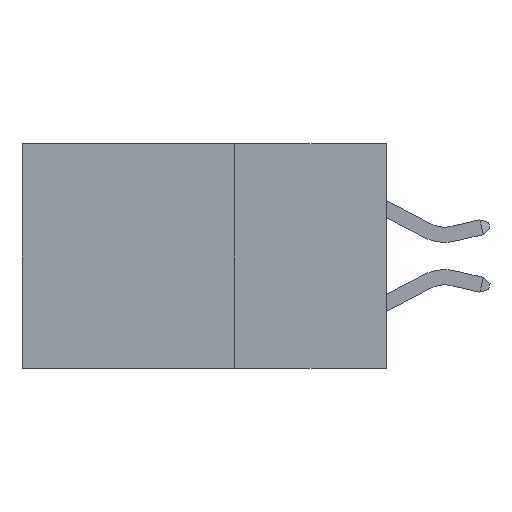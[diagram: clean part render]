
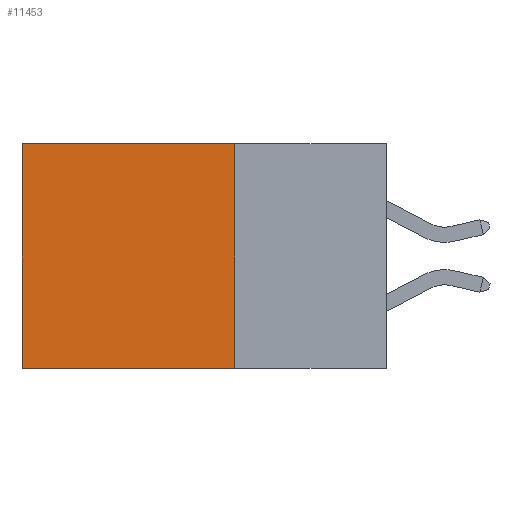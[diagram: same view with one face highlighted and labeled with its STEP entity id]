
A CAD part, left-side view. The second image highlights one B-rep face of the part: STEP entity #11453.
In plain terms, the highlighted planar face has unit normal (-1, 0, 0).
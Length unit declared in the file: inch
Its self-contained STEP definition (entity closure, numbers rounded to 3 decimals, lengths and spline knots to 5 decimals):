
#106 = DIRECTION ( 'NONE',  ( 0., 1., 0. ) ) ;
#119 = CARTESIAN_POINT ( 'NONE',  ( 0.2615, 0.25, -0.37 ) ) ;
#331 = ORIENTED_EDGE ( 'NONE', *, *, #10118, .F. ) ;
#412 = DIRECTION ( 'NONE',  ( 0., 1., 0. ) ) ;
#419 = CARTESIAN_POINT ( 'NONE',  ( 0.2615, 0.25, 0. ) ) ;
#1147 = VECTOR ( 'NONE', #9202, 39.37008 ) ;
#1155 = ORIENTED_EDGE ( 'NONE', *, *, #8568, .F. ) ;
#1215 = CARTESIAN_POINT ( 'NONE',  ( 0.2615, 0.6, -0.37 ) ) ;
#2451 = EDGE_LOOP ( 'NONE', ( #2578, #1155, #331, #12251 ) ) ;
#2578 = ORIENTED_EDGE ( 'NONE', *, *, #10902, .T. ) ;
#3011 = LINE ( 'NONE', #3895, #10231 ) ;
#3575 = DIRECTION ( 'NONE',  ( 0., 0., -1. ) ) ;
#3837 = LINE ( 'NONE', #119, #11306 ) ;
#3895 = CARTESIAN_POINT ( 'NONE',  ( 0.2615, 0.6, -0.37 ) ) ;
#4737 = EDGE_CURVE ( 'NONE', #6870, #5775, #8272, .T. ) ;
#5775 = VERTEX_POINT ( 'NONE', #8437 ) ;
#6484 = VERTEX_POINT ( 'NONE', #11550 ) ;
#6870 = VERTEX_POINT ( 'NONE', #9332 ) ;
#7718 = FACE_OUTER_BOUND ( 'NONE', #2451, .T. ) ;
#8272 = LINE ( 'NONE', #419, #10772 ) ;
#8421 = VERTEX_POINT ( 'NONE', #1215 ) ;
#8437 = CARTESIAN_POINT ( 'NONE',  ( 0.2615, 0.6, 0. ) ) ;
#8568 = EDGE_CURVE ( 'NONE', #6484, #8421, #3837, .T. ) ;
#8792 = LINE ( 'NONE', #9743, #1147 ) ;
#9202 = DIRECTION ( 'NONE',  ( 0., 0., -1. ) ) ;
#9332 = CARTESIAN_POINT ( 'NONE',  ( 0.2615, 0.25, 0. ) ) ;
#9339 = DIRECTION ( 'NONE',  ( 0., 0., -1. ) ) ;
#9365 = DIRECTION ( 'NONE',  ( 1., 0., 0. ) ) ;
#9427 = CARTESIAN_POINT ( 'NONE',  ( 0.2615, 0.25, -0.37 ) ) ;
#9598 = PLANE ( 'NONE',  #9878 ) ;
#9743 = CARTESIAN_POINT ( 'NONE',  ( 0.2615, 0.25, -0.37 ) ) ;
#9878 = AXIS2_PLACEMENT_3D ( 'NONE', #9427, #9365, #9339 ) ;
#10118 = EDGE_CURVE ( 'NONE', #6870, #6484, #8792, .T. ) ;
#10231 = VECTOR ( 'NONE', #3575, 39.37008 ) ;
#10772 = VECTOR ( 'NONE', #412, 39.37008 ) ;
#10902 = EDGE_CURVE ( 'NONE', #5775, #8421, #3011, .T. ) ;
#11306 = VECTOR ( 'NONE', #106, 39.37008 ) ;
#11453 = ADVANCED_FACE ( 'NONE', ( #7718 ), #9598, .F. ) ;
#11550 = CARTESIAN_POINT ( 'NONE',  ( 0.2615, 0.25, -0.37 ) ) ;
#12251 = ORIENTED_EDGE ( 'NONE', *, *, #4737, .T. ) ;
